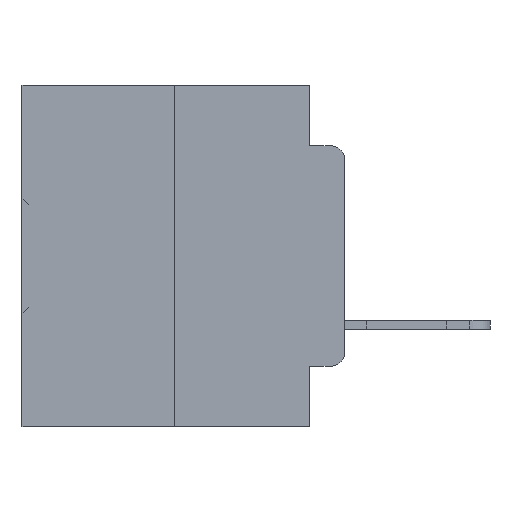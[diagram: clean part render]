
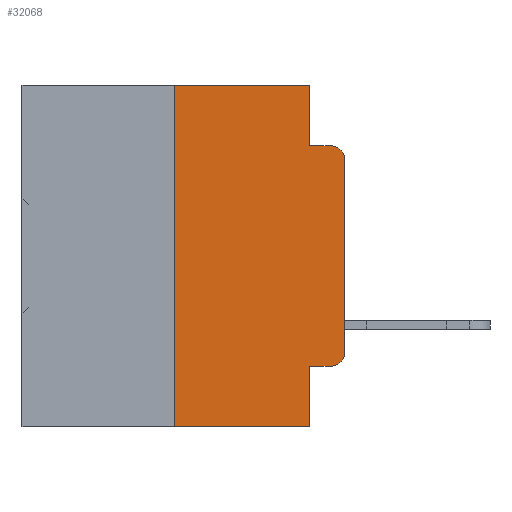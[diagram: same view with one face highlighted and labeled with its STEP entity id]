
A CAD part, left-side view. The second image highlights one B-rep face of the part: STEP entity #32068.
In plain terms, the highlighted planar face has unit normal (-1, 0, 0).
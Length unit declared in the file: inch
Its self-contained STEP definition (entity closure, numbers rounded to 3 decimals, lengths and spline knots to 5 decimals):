
#2061 = VECTOR ( 'NONE', #17754, 39.37008 ) ;
#2111 = EDGE_CURVE ( 'NONE', #19971, #11556, #11658, .T. ) ;
#2114 = DIRECTION ( 'NONE',  ( 0., -1., 0. ) ) ;
#2173 = EDGE_CURVE ( 'NONE', #11556, #8463, #36840, .T. ) ;
#2565 = VERTEX_POINT ( 'NONE', #36679 ) ;
#2649 = DIRECTION ( 'NONE',  ( 0., 0., -1. ) ) ;
#2745 = DIRECTION ( 'NONE',  ( 0., 0., -1. ) ) ;
#2797 = DIRECTION ( 'NONE',  ( -1., 0., 0. ) ) ;
#2923 = CARTESIAN_POINT ( 'NONE',  ( 0., 0.02, -0.1085 ) ) ;
#2925 = CARTESIAN_POINT ( 'NONE',  ( 0., 0.051, 0. ) ) ;
#3495 = ORIENTED_EDGE ( 'NONE', *, *, #2173, .F. ) ;
#4119 = VECTOR ( 'NONE', #2114, 39.37008 ) ;
#4249 = CARTESIAN_POINT ( 'NONE',  ( 0., 0.051, -0.0885 ) ) ;
#4485 = EDGE_CURVE ( 'NONE', #13704, #2565, #31991, .T. ) ;
#4500 = VERTEX_POINT ( 'NONE', #17536 ) ;
#4537 = ORIENTED_EDGE ( 'NONE', *, *, #20354, .F. ) ;
#4821 = LINE ( 'NONE', #24399, #19428 ) ;
#4972 = ORIENTED_EDGE ( 'NONE', *, *, #17075, .T. ) ;
#5978 = ORIENTED_EDGE ( 'NONE', *, *, #28933, .T. ) ;
#8463 = VERTEX_POINT ( 'NONE', #2925 ) ;
#9448 = CARTESIAN_POINT ( 'NONE',  ( 0., 0.473, -0.5 ) ) ;
#9478 = DIRECTION ( 'NONE',  ( 0., -1., 0. ) ) ;
#9925 = EDGE_CURVE ( 'NONE', #9996, #29021, #21333, .T. ) ;
#9996 = VERTEX_POINT ( 'NONE', #32442 ) ;
#10240 = DIRECTION ( 'NONE',  ( 0., -1., 0. ) ) ;
#10836 = EDGE_LOOP ( 'NONE', ( #17197, #14056, #15358, #20046, #3495, #29771, #4972, #4537, #5978, #10885 ) ) ;
#10885 = ORIENTED_EDGE ( 'NONE', *, *, #4485, .T. ) ;
#11034 = LINE ( 'NONE', #14929, #2061 ) ;
#11556 = VERTEX_POINT ( 'NONE', #13242 ) ;
#11631 = PLANE ( 'NONE',  #32816 ) ;
#11658 = LINE ( 'NONE', #15833, #31381 ) ;
#12069 = LINE ( 'NONE', #19741, #4119 ) ;
#12768 = VECTOR ( 'NONE', #35894, 39.37008 ) ;
#13069 = AXIS2_PLACEMENT_3D ( 'NONE', #15846, #15752, #15704 ) ;
#13242 = CARTESIAN_POINT ( 'NONE',  ( 0., 0.25, 0. ) ) ;
#13659 = VECTOR ( 'NONE', #23260, 39.37008 ) ;
#13677 = LINE ( 'NONE', #27921, #12768 ) ;
#13704 = VERTEX_POINT ( 'NONE', #32111 ) ;
#14056 = ORIENTED_EDGE ( 'NONE', *, *, #9925, .T. ) ;
#14802 = VECTOR ( 'NONE', #36899, 39.37008 ) ;
#14929 = CARTESIAN_POINT ( 'NONE',  ( 0., 0., 0. ) ) ;
#15358 = ORIENTED_EDGE ( 'NONE', *, *, #22660, .F. ) ;
#15658 = DIRECTION ( 'NONE',  ( 0., 0., 1. ) ) ;
#15704 = DIRECTION ( 'NONE',  ( 0., 0., -1. ) ) ;
#15752 = DIRECTION ( 'NONE',  ( -1., 0., 0. ) ) ;
#15833 = CARTESIAN_POINT ( 'NONE',  ( 0., 0.25, 0. ) ) ;
#15846 = CARTESIAN_POINT ( 'NONE',  ( 0., 0.02, -0.3915 ) ) ;
#17075 = EDGE_CURVE ( 'NONE', #19971, #27400, #26147, .T. ) ;
#17197 = ORIENTED_EDGE ( 'NONE', *, *, #30260, .T. ) ;
#17536 = CARTESIAN_POINT ( 'NONE',  ( 0., 0.051, -0.4115 ) ) ;
#17677 = AXIS2_PLACEMENT_3D ( 'NONE', #2923, #2797, #2745 ) ;
#17754 = DIRECTION ( 'NONE',  ( 0., 0., 1. ) ) ;
#19428 = VECTOR ( 'NONE', #10240, 39.37008 ) ;
#19741 = CARTESIAN_POINT ( 'NONE',  ( 0., 0.051, -0.4115 ) ) ;
#19971 = VERTEX_POINT ( 'NONE', #31668 ) ;
#20046 = ORIENTED_EDGE ( 'NONE', *, *, #34144, .F. ) ;
#20253 = DIRECTION ( 'NONE',  ( 1., 0., 0. ) ) ;
#20354 = EDGE_CURVE ( 'NONE', #4500, #27400, #13677, .T. ) ;
#20474 = CARTESIAN_POINT ( 'NONE',  ( 0., 0.051, 0. ) ) ;
#21333 = CIRCLE ( 'NONE', #17677, 0.02 ) ;
#22660 = EDGE_CURVE ( 'NONE', #23826, #29021, #4821, .T. ) ;
#23260 = DIRECTION ( 'NONE',  ( 0., 0., -1. ) ) ;
#23826 = VERTEX_POINT ( 'NONE', #4249 ) ;
#24399 = CARTESIAN_POINT ( 'NONE',  ( 0., 0.051, -0.0885 ) ) ;
#26147 = LINE ( 'NONE', #9448, #32592 ) ;
#26342 = FACE_OUTER_BOUND ( 'NONE', #10836, .T. ) ;
#27400 = VERTEX_POINT ( 'NONE', #33593 ) ;
#27921 = CARTESIAN_POINT ( 'NONE',  ( 0., 0.051, 0. ) ) ;
#28493 = CARTESIAN_POINT ( 'NONE',  ( 0., 0.473, 0. ) ) ;
#28933 = EDGE_CURVE ( 'NONE', #4500, #13704, #12069, .T. ) ;
#29021 = VERTEX_POINT ( 'NONE', #33943 ) ;
#29771 = ORIENTED_EDGE ( 'NONE', *, *, #2111, .F. ) ;
#30260 = EDGE_CURVE ( 'NONE', #2565, #9996, #11034, .T. ) ;
#31381 = VECTOR ( 'NONE', #15658, 39.37008 ) ;
#31668 = CARTESIAN_POINT ( 'NONE',  ( 0., 0.25, -0.5 ) ) ;
#31991 = CIRCLE ( 'NONE', #13069, 0.02 ) ;
#32068 = ADVANCED_FACE ( 'NONE', ( #26342 ), #11631, .F. ) ;
#32111 = CARTESIAN_POINT ( 'NONE',  ( 0., 0.02, -0.4115 ) ) ;
#32442 = CARTESIAN_POINT ( 'NONE',  ( 0., 0., -0.1085 ) ) ;
#32592 = VECTOR ( 'NONE', #9478, 39.37008 ) ;
#32816 = AXIS2_PLACEMENT_3D ( 'NONE', #28493, #20253, #2649 ) ;
#33593 = CARTESIAN_POINT ( 'NONE',  ( 0., 0.051, -0.5 ) ) ;
#33943 = CARTESIAN_POINT ( 'NONE',  ( 0., 0.02, -0.0885 ) ) ;
#34144 = EDGE_CURVE ( 'NONE', #8463, #23826, #35789, .T. ) ;
#35789 = LINE ( 'NONE', #20474, #13659 ) ;
#35894 = DIRECTION ( 'NONE',  ( 0., 0., -1. ) ) ;
#36595 = CARTESIAN_POINT ( 'NONE',  ( 0., 0.473, 0. ) ) ;
#36679 = CARTESIAN_POINT ( 'NONE',  ( 0., 0., -0.3915 ) ) ;
#36840 = LINE ( 'NONE', #36595, #14802 ) ;
#36899 = DIRECTION ( 'NONE',  ( 0., -1., 0. ) ) ;
